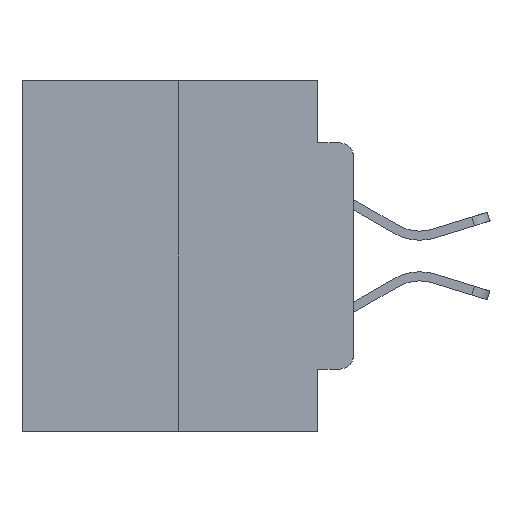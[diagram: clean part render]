
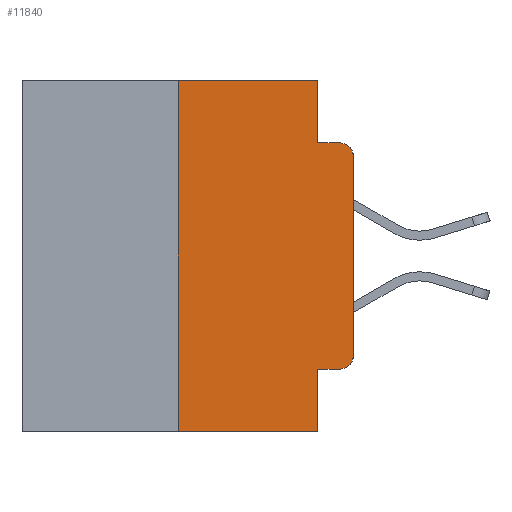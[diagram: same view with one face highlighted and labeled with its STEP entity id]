
A CAD part, left-side view. The second image highlights one B-rep face of the part: STEP entity #11840.
In plain terms, the highlighted planar face has unit normal (-1, 0, 0).
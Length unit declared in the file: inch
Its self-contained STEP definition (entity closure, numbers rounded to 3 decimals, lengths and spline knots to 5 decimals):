
#80 = CARTESIAN_POINT ( 'NONE',  ( 0., 0.25, 0. ) ) ;
#108 = ORIENTED_EDGE ( 'NONE', *, *, #18105, .T. ) ;
#236 = ORIENTED_EDGE ( 'NONE', *, *, #20420, .F. ) ;
#265 = LINE ( 'NONE', #22498, #4658 ) ;
#284 = VERTEX_POINT ( 'NONE', #20033 ) ;
#434 = LINE ( 'NONE', #20719, #4821 ) ;
#561 = DIRECTION ( 'NONE',  ( 0., -1., 0. ) ) ;
#837 = VERTEX_POINT ( 'NONE', #22158 ) ;
#1316 = CARTESIAN_POINT ( 'NONE',  ( 0., 0.051, -0.4115 ) ) ;
#1397 = VECTOR ( 'NONE', #14100, 39.37008 ) ;
#1841 = EDGE_CURVE ( 'NONE', #13279, #3502, #8261, .T. ) ;
#2285 = VERTEX_POINT ( 'NONE', #12507 ) ;
#2841 = ORIENTED_EDGE ( 'NONE', *, *, #1841, .F. ) ;
#2962 = ORIENTED_EDGE ( 'NONE', *, *, #8026, .F. ) ;
#3077 = DIRECTION ( 'NONE',  ( -1., 0., 0. ) ) ;
#3502 = VERTEX_POINT ( 'NONE', #16291 ) ;
#3582 = ORIENTED_EDGE ( 'NONE', *, *, #18202, .T. ) ;
#4407 = ORIENTED_EDGE ( 'NONE', *, *, #24442, .T. ) ;
#4644 = LINE ( 'NONE', #80, #25177 ) ;
#4658 = VECTOR ( 'NONE', #8270, 39.37008 ) ;
#4660 = EDGE_CURVE ( 'NONE', #17324, #16544, #18084, .T. ) ;
#4821 = VECTOR ( 'NONE', #12526, 39.37008 ) ;
#5638 = CARTESIAN_POINT ( 'NONE',  ( 0., 0.25, 0. ) ) ;
#6746 = ORIENTED_EDGE ( 'NONE', *, *, #17699, .F. ) ;
#7130 = DIRECTION ( 'NONE',  ( -1., 0., 0. ) ) ;
#7370 = CARTESIAN_POINT ( 'NONE',  ( 0., 0.473, 0. ) ) ;
#7684 = CARTESIAN_POINT ( 'NONE',  ( 0., 0.051, -0.5 ) ) ;
#7763 = CIRCLE ( 'NONE', #20827, 0.02 ) ;
#7812 = CARTESIAN_POINT ( 'NONE',  ( 0., 0., 0. ) ) ;
#8026 = EDGE_CURVE ( 'NONE', #2285, #13279, #4644, .T. ) ;
#8261 = LINE ( 'NONE', #23271, #13153 ) ;
#8270 = DIRECTION ( 'NONE',  ( 0., 0., -1. ) ) ;
#8302 = ORIENTED_EDGE ( 'NONE', *, *, #4660, .T. ) ;
#9476 = DIRECTION ( 'NONE',  ( 1., 0., 0. ) ) ;
#9895 = DIRECTION ( 'NONE',  ( 0., -1., 0. ) ) ;
#9912 = ORIENTED_EDGE ( 'NONE', *, *, #26225, .F. ) ;
#10187 = CIRCLE ( 'NONE', #20317, 0.02 ) ;
#11501 = CARTESIAN_POINT ( 'NONE',  ( 0., 0.473, -0.5 ) ) ;
#11840 = ADVANCED_FACE ( 'NONE', ( #17850 ), #19689, .F. ) ;
#12122 = VECTOR ( 'NONE', #23682, 39.37008 ) ;
#12345 = CARTESIAN_POINT ( 'NONE',  ( 0., 0.051, 0. ) ) ;
#12507 = CARTESIAN_POINT ( 'NONE',  ( 0., 0.25, -0.5 ) ) ;
#12526 = DIRECTION ( 'NONE',  ( 0., -1., 0. ) ) ;
#12949 = CARTESIAN_POINT ( 'NONE',  ( 0., 0., -0.1085 ) ) ;
#13153 = VECTOR ( 'NONE', #561, 39.37008 ) ;
#13279 = VERTEX_POINT ( 'NONE', #5638 ) ;
#13803 = VECTOR ( 'NONE', #9895, 39.37008 ) ;
#14100 = DIRECTION ( 'NONE',  ( 0., 0., 1. ) ) ;
#14099 = VECTOR ( 'NONE', #24394, 39.37008 ) ;
#14118 = EDGE_CURVE ( 'NONE', #837, #17324, #7763, .T. ) ;
#15148 = CARTESIAN_POINT ( 'NONE',  ( 0., 0.02, -0.0885 ) ) ;
#15658 = CARTESIAN_POINT ( 'NONE',  ( 0., 0.02, -0.1085 ) ) ;
#16291 = CARTESIAN_POINT ( 'NONE',  ( 0., 0.051, 0. ) ) ;
#16544 = VERTEX_POINT ( 'NONE', #12949 ) ;
#17324 = VERTEX_POINT ( 'NONE', #17396 ) ;
#17396 = CARTESIAN_POINT ( 'NONE',  ( 0., 0., -0.3915 ) ) ;
#17681 = DIRECTION ( 'NONE',  ( 0., 0., -1. ) ) ;
#17699 = EDGE_CURVE ( 'NONE', #3502, #21578, #265, .T. ) ;
#17850 = FACE_OUTER_BOUND ( 'NONE', #24912, .T. ) ;
#18084 = LINE ( 'NONE', #7812, #1397 ) ;
#18105 = EDGE_CURVE ( 'NONE', #2285, #20181, #22950, .T. ) ;
#18202 = EDGE_CURVE ( 'NONE', #284, #837, #24550, .T. ) ;
#18412 = CARTESIAN_POINT ( 'NONE',  ( 0., 0.051, -0.0885 ) ) ;
#18892 = ORIENTED_EDGE ( 'NONE', *, *, #14118, .T. ) ;
#18950 = DIRECTION ( 'NONE',  ( 0., 0., 1. ) ) ;
#19462 = CARTESIAN_POINT ( 'NONE',  ( 0., 0.02, -0.3915 ) ) ;
#19505 = LINE ( 'NONE', #12345, #14099 ) ;
#19689 = PLANE ( 'NONE',  #22141 ) ;
#20033 = CARTESIAN_POINT ( 'NONE',  ( 0., 0.051, -0.4115 ) ) ;
#20181 = VERTEX_POINT ( 'NONE', #7684 ) ;
#20317 = AXIS2_PLACEMENT_3D ( 'NONE', #15658, #3077, #17681 ) ;
#20420 = EDGE_CURVE ( 'NONE', #21578, #21810, #434, .T. ) ;
#20719 = CARTESIAN_POINT ( 'NONE',  ( 0., 0.051, -0.0885 ) ) ;
#20827 = AXIS2_PLACEMENT_3D ( 'NONE', #19462, #7130, #21509 ) ;
#21509 = DIRECTION ( 'NONE',  ( 0., 0., -1. ) ) ;
#21578 = VERTEX_POINT ( 'NONE', #18412 ) ;
#21810 = VERTEX_POINT ( 'NONE', #15148 ) ;
#22141 = AXIS2_PLACEMENT_3D ( 'NONE', #7370, #9476, #23743 ) ;
#22158 = CARTESIAN_POINT ( 'NONE',  ( 0., 0.02, -0.4115 ) ) ;
#22498 = CARTESIAN_POINT ( 'NONE',  ( 0., 0.051, 0. ) ) ;
#22950 = LINE ( 'NONE', #11501, #12122 ) ;
#23271 = CARTESIAN_POINT ( 'NONE',  ( 0., 0.473, 0. ) ) ;
#23682 = DIRECTION ( 'NONE',  ( 0., -1., 0. ) ) ;
#23743 = DIRECTION ( 'NONE',  ( 0., 0., -1. ) ) ;
#24394 = DIRECTION ( 'NONE',  ( 0., 0., -1. ) ) ;
#24442 = EDGE_CURVE ( 'NONE', #16544, #21810, #10187, .T. ) ;
#24550 = LINE ( 'NONE', #1316, #13803 ) ;
#24912 = EDGE_LOOP ( 'NONE', ( #8302, #4407, #236, #6746, #2841, #2962, #108, #9912, #3582, #18892 ) ) ;
#25177 = VECTOR ( 'NONE', #18950, 39.37008 ) ;
#26225 = EDGE_CURVE ( 'NONE', #284, #20181, #19505, .T. ) ;
